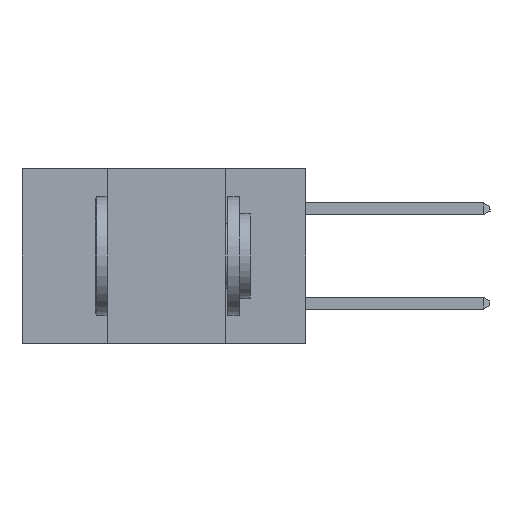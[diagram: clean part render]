
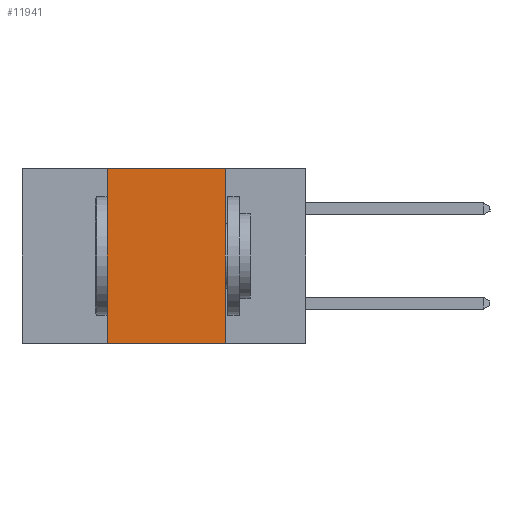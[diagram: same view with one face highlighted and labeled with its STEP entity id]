
A CAD part, left-side view. The second image highlights one B-rep face of the part: STEP entity #11941.
In plain terms, the highlighted planar face has unit normal (-1, 0, 0).
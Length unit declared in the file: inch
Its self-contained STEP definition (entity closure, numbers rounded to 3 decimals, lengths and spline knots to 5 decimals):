
#430 = FACE_OUTER_BOUND ( 'NONE', #13629, .T. ) ;
#524 = ORIENTED_EDGE ( 'NONE', *, *, #23163, .F. ) ;
#927 = CARTESIAN_POINT ( 'NONE',  ( 0., 0.6, -0.37 ) ) ;
#1728 = CARTESIAN_POINT ( 'NONE',  ( 0., 0.42, -0.37 ) ) ;
#2039 = VERTEX_POINT ( 'NONE', #24012 ) ;
#3293 = EDGE_CURVE ( 'NONE', #24112, #17961, #11992, .T. ) ;
#3548 = VECTOR ( 'NONE', #23387, 39.37008 ) ;
#4222 = LINE ( 'NONE', #21420, #3548 ) ;
#4940 = VECTOR ( 'NONE', #6944, 39.37008 ) ;
#6944 = DIRECTION ( 'NONE',  ( 0., 0., 1. ) ) ;
#7508 = EDGE_CURVE ( 'NONE', #24112, #2039, #15811, .T. ) ;
#7575 = DIRECTION ( 'NONE',  ( 1., 0., 0. ) ) ;
#7819 = LINE ( 'NONE', #23860, #17938 ) ;
#8852 = EDGE_CURVE ( 'NONE', #13037, #17961, #4222, .T. ) ;
#9799 = ORIENTED_EDGE ( 'NONE', *, *, #7508, .F. ) ;
#11364 = VECTOR ( 'NONE', #17161, 39.37008 ) ;
#11941 = ADVANCED_FACE ( 'NONE', ( #430 ), #13581, .F. ) ;
#11992 = LINE ( 'NONE', #927, #11364 ) ;
#12961 = ORIENTED_EDGE ( 'NONE', *, *, #3293, .T. ) ;
#13037 = VERTEX_POINT ( 'NONE', #20572 ) ;
#13581 = PLANE ( 'NONE',  #13838 ) ;
#13629 = EDGE_LOOP ( 'NONE', ( #23470, #524, #9799, #12961 ) ) ;
#13838 = AXIS2_PLACEMENT_3D ( 'NONE', #21574, #7575, #21670 ) ;
#15811 = LINE ( 'NONE', #17026, #4940 ) ;
#16942 = CARTESIAN_POINT ( 'NONE',  ( 0., 0.17, -0.37 ) ) ;
#17026 = CARTESIAN_POINT ( 'NONE',  ( 0., 0.42, 0. ) ) ;
#17161 = DIRECTION ( 'NONE',  ( 0., -1., 0. ) ) ;
#17938 = VECTOR ( 'NONE', #25827, 39.37008 ) ;
#17961 = VERTEX_POINT ( 'NONE', #16942 ) ;
#20572 = CARTESIAN_POINT ( 'NONE',  ( 0., 0.17, 0. ) ) ;
#21420 = CARTESIAN_POINT ( 'NONE',  ( 0., 0.17, 0. ) ) ;
#21574 = CARTESIAN_POINT ( 'NONE',  ( 0., 0.6, 0. ) ) ;
#21670 = DIRECTION ( 'NONE',  ( 0., 0., -1. ) ) ;
#23163 = EDGE_CURVE ( 'NONE', #2039, #13037, #7819, .T. ) ;
#23387 = DIRECTION ( 'NONE',  ( 0., 0., -1. ) ) ;
#23470 = ORIENTED_EDGE ( 'NONE', *, *, #8852, .F. ) ;
#23860 = CARTESIAN_POINT ( 'NONE',  ( 0., 0.6, 0. ) ) ;
#24012 = CARTESIAN_POINT ( 'NONE',  ( 0., 0.42, 0. ) ) ;
#24112 = VERTEX_POINT ( 'NONE', #1728 ) ;
#25827 = DIRECTION ( 'NONE',  ( 0., -1., 0. ) ) ;
